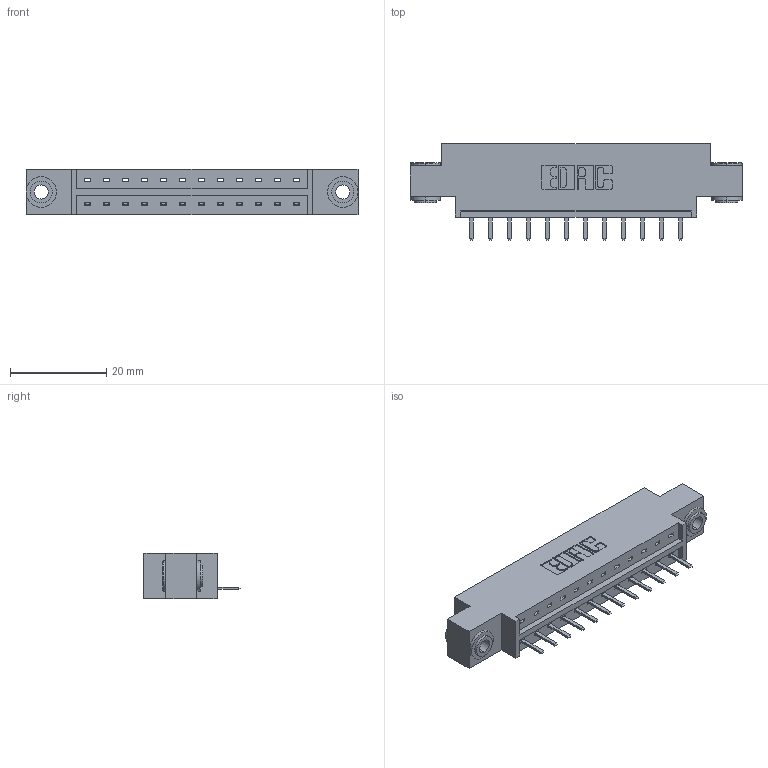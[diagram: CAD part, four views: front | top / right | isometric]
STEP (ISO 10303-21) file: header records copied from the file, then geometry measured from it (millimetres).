
FILE_DESCRIPTION (( 'STEP AP203' ), '1' );
FILE_NAME ('333-012-520-603.STEP', '2018-07-31T23:54:52', ( '' ), ( '' ), 'SwSTEP 2.0', 'SolidWorks 2016', '' );
FILE_SCHEMA (( 'CONFIG_CONTROL_DESIGN' ));
Length unit declared in the file: inch
Products named in the file (4): 333-012-520-603; 333 Part_Offset - .156 Dia - TH; 345-292-001_345-293-120; 345-250-002_345-250-002-102
Assembly tree (15 placements, depth 2):
  333-012-520-603
    333 Part_Offset - .156 Dia - TH
    345-292-001_345-293-120  x12
    345-250-002_345-250-002-102  x2
Bounding box: 69.09 x 20.02 x 9.4 mm (x, y, z)
Volume: 6451.3 mm3; surface area: 7088.3 mm2
Topology: 15 solids, 15 shells, 900 faces, 2607 edges, 1702 vertices
Faces by surface type: plane 612, cylinder 280, cone 8
Entity records: 12112 total; most frequent: CARTESIAN_POINT 2085, ORIENTED_EDGE 2014, DIRECTION 1841, EDGE_CURVE 1007, LINE 851, VECTOR 851, VERTEX_POINT 666, AXIS2_PLACEMENT_3D 495
